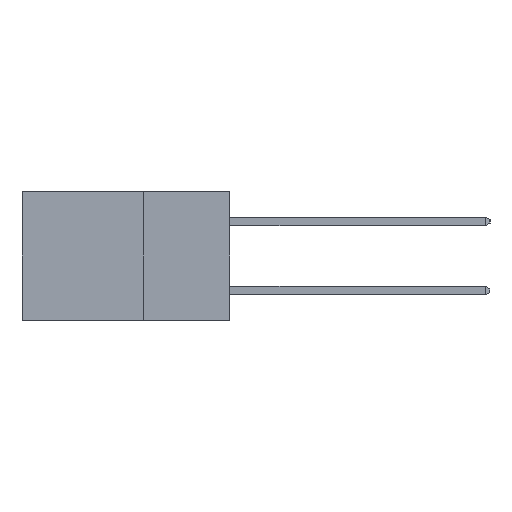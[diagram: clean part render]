
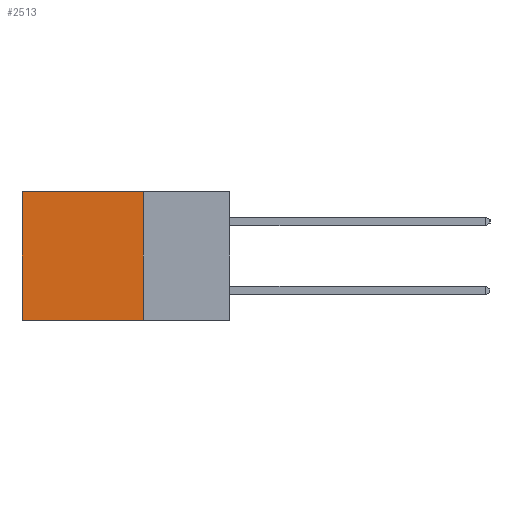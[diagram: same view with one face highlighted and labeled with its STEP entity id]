
A CAD part, left-side view. The second image highlights one B-rep face of the part: STEP entity #2513.
In plain terms, the highlighted planar face has unit normal (-1, 0, 0).
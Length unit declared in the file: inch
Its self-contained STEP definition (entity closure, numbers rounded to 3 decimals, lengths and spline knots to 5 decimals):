
#194 = EDGE_CURVE ( 'NONE', #12920, #11332, #8506, .T. ) ;
#256 = VECTOR ( 'NONE', #779, 39.37008 ) ;
#335 = CARTESIAN_POINT ( 'NONE',  ( 0.298, 0.6, 0. ) ) ;
#501 = DIRECTION ( 'NONE',  ( 0., 0., -1. ) ) ;
#779 = DIRECTION ( 'NONE',  ( 0., 0., -1. ) ) ;
#1355 = FACE_OUTER_BOUND ( 'NONE', #16516, .T. ) ;
#1812 = LINE ( 'NONE', #1831, #10767 ) ;
#1831 = CARTESIAN_POINT ( 'NONE',  ( 0.298, 0.25, -0.37 ) ) ;
#1996 = PLANE ( 'NONE',  #16105 ) ;
#2513 = ADVANCED_FACE ( 'NONE', ( #1355 ), #1996, .F. ) ;
#3000 = ORIENTED_EDGE ( 'NONE', *, *, #194, .T. ) ;
#3398 = ORIENTED_EDGE ( 'NONE', *, *, #21382, .F. ) ;
#3518 = CARTESIAN_POINT ( 'NONE',  ( 0.298, 0.25, 0. ) ) ;
#3802 = VECTOR ( 'NONE', #10840, 39.37008 ) ;
#5192 = CARTESIAN_POINT ( 'NONE',  ( 0.298, 0.25, 0. ) ) ;
#5444 = EDGE_CURVE ( 'NONE', #11332, #12493, #6040, .T. ) ;
#6040 = LINE ( 'NONE', #335, #16047 ) ;
#6273 = DIRECTION ( 'NONE',  ( 0., 0., -1. ) ) ;
#8506 = LINE ( 'NONE', #21772, #3802 ) ;
#9859 = EDGE_CURVE ( 'NONE', #18984, #12493, #1812, .T. ) ;
#10767 = VECTOR ( 'NONE', #21574, 39.37008 ) ;
#10840 = DIRECTION ( 'NONE',  ( 0., 1., 0. ) ) ;
#11332 = VERTEX_POINT ( 'NONE', #20673 ) ;
#12493 = VERTEX_POINT ( 'NONE', #22033 ) ;
#12920 = VERTEX_POINT ( 'NONE', #5192 ) ;
#14102 = ORIENTED_EDGE ( 'NONE', *, *, #5444, .T. ) ;
#14579 = LINE ( 'NONE', #22356, #256 ) ;
#16047 = VECTOR ( 'NONE', #501, 39.37008 ) ;
#16105 = AXIS2_PLACEMENT_3D ( 'NONE', #3518, #18303, #6273 ) ;
#16516 = EDGE_LOOP ( 'NONE', ( #14102, #20112, #3398, #3000 ) ) ;
#18303 = DIRECTION ( 'NONE',  ( 1., 0., 0. ) ) ;
#18984 = VERTEX_POINT ( 'NONE', #20841 ) ;
#20112 = ORIENTED_EDGE ( 'NONE', *, *, #9859, .F. ) ;
#20673 = CARTESIAN_POINT ( 'NONE',  ( 0.298, 0.6, 0. ) ) ;
#20841 = CARTESIAN_POINT ( 'NONE',  ( 0.298, 0.25, -0.37 ) ) ;
#21382 = EDGE_CURVE ( 'NONE', #12920, #18984, #14579, .T. ) ;
#21574 = DIRECTION ( 'NONE',  ( 0., 1., 0. ) ) ;
#21772 = CARTESIAN_POINT ( 'NONE',  ( 0.298, 0.25, 0. ) ) ;
#22033 = CARTESIAN_POINT ( 'NONE',  ( 0.298, 0.6, -0.37 ) ) ;
#22356 = CARTESIAN_POINT ( 'NONE',  ( 0.298, 0.25, 0. ) ) ;
